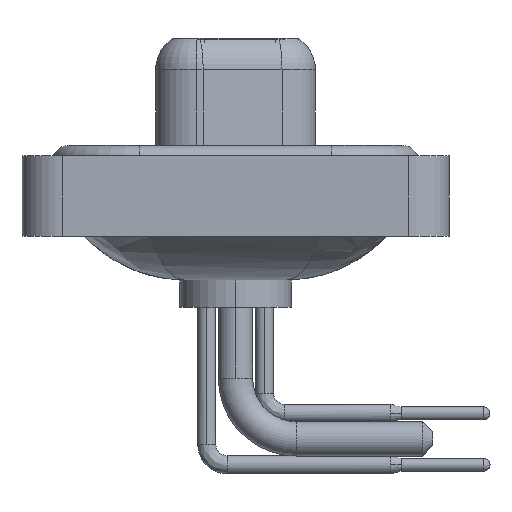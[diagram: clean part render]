
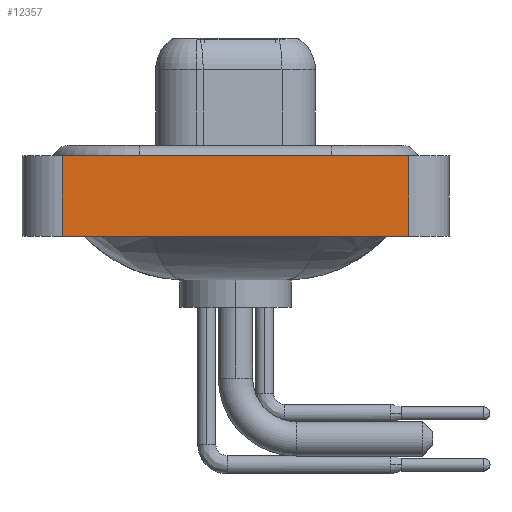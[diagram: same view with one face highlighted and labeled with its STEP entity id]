
A CAD part, left-side view. The second image highlights one B-rep face of the part: STEP entity #12357.
In plain terms, the highlighted planar face has unit normal (-1, 0, 0).
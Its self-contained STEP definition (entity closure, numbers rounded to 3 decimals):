
#54 = AXIS2_PLACEMENT_3D ( 'NONE', #13500, #13397, #5321 ) ;
#2342 = PLANE ( 'NONE',  #54 ) ;
#2383 = EDGE_CURVE ( 'NONE', #3965, #18812, #11058, .T. ) ;
#3566 = VECTOR ( 'NONE', #17792, 1000. ) ;
#3796 = VERTEX_POINT ( 'NONE', #17545 ) ;
#3965 = VERTEX_POINT ( 'NONE', #13707 ) ;
#5321 = DIRECTION ( 'NONE',  ( 0., 0., 1. ) ) ;
#5800 = VECTOR ( 'NONE', #6277, 1000. ) ;
#5922 = EDGE_CURVE ( 'NONE', #18812, #3796, #17888, .T. ) ;
#6277 = DIRECTION ( 'NONE',  ( 0., -1., 0. ) ) ;
#6497 = CARTESIAN_POINT ( 'NONE',  ( -7.35, 8.55, 0.4 ) ) ;
#6571 = LINE ( 'NONE', #8274, #5800 ) ;
#6676 = ORIENTED_EDGE ( 'NONE', *, *, #2383, .T. ) ;
#7340 = EDGE_CURVE ( 'NONE', #3965, #14514, #11028, .T. ) ;
#8274 = CARTESIAN_POINT ( 'NONE',  ( -7.35, -8.55, 0.4 ) ) ;
#9694 = CARTESIAN_POINT ( 'NONE',  ( -7.35, -8.55, -3.6 ) ) ;
#10178 = CARTESIAN_POINT ( 'NONE',  ( -7.35, -8.55, -3.6 ) ) ;
#11028 = LINE ( 'NONE', #20796, #20215 ) ;
#11058 = LINE ( 'NONE', #15845, #17326 ) ;
#11278 = ORIENTED_EDGE ( 'NONE', *, *, #5922, .T. ) ;
#12357 = ADVANCED_FACE ( 'NONE', ( #13608 ), #2342, .T. ) ;
#12728 = DIRECTION ( 'NONE',  ( 0., 0., 1. ) ) ;
#13397 = DIRECTION ( 'NONE',  ( -1., 0., 0. ) ) ;
#13500 = CARTESIAN_POINT ( 'NONE',  ( -7.35, -8.55, -3.6 ) ) ;
#13608 = FACE_OUTER_BOUND ( 'NONE', #17382, .T. ) ;
#13707 = CARTESIAN_POINT ( 'NONE',  ( -7.35, 8.55, -3.6 ) ) ;
#14271 = ORIENTED_EDGE ( 'NONE', *, *, #7340, .F. ) ;
#14514 = VERTEX_POINT ( 'NONE', #6497 ) ;
#15845 = CARTESIAN_POINT ( 'NONE',  ( -7.35, -8.55, -3.6 ) ) ;
#17326 = VECTOR ( 'NONE', #17542, 1000. ) ;
#17382 = EDGE_LOOP ( 'NONE', ( #11278, #17510, #14271, #6676 ) ) ;
#17510 = ORIENTED_EDGE ( 'NONE', *, *, #20029, .F. ) ;
#17542 = DIRECTION ( 'NONE',  ( 0., -1., 0. ) ) ;
#17545 = CARTESIAN_POINT ( 'NONE',  ( -7.35, -8.55, 0.4 ) ) ;
#17792 = DIRECTION ( 'NONE',  ( 0., 0., 1. ) ) ;
#17888 = LINE ( 'NONE', #9694, #3566 ) ;
#18812 = VERTEX_POINT ( 'NONE', #10178 ) ;
#20029 = EDGE_CURVE ( 'NONE', #14514, #3796, #6571, .T. ) ;
#20215 = VECTOR ( 'NONE', #12728, 1000. ) ;
#20796 = CARTESIAN_POINT ( 'NONE',  ( -7.35, 8.55, -3.6 ) ) ;
